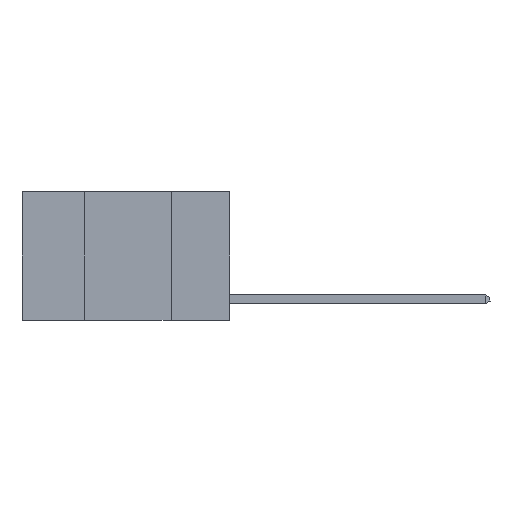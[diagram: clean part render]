
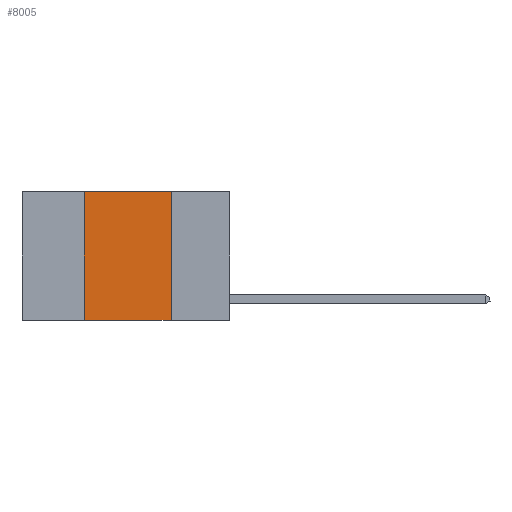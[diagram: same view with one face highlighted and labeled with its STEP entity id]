
A CAD part, left-side view. The second image highlights one B-rep face of the part: STEP entity #8005.
In plain terms, the highlighted planar face has unit normal (-1, 0, 0).
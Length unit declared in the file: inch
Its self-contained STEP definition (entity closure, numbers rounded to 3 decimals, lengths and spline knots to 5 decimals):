
#105 = CARTESIAN_POINT ( 'NONE',  ( 0., 0.6, -0.37 ) ) ;
#551 = CARTESIAN_POINT ( 'NONE',  ( 0., 0.42, -0.37 ) ) ;
#796 = CARTESIAN_POINT ( 'NONE',  ( 0., 0.6, 0. ) ) ;
#1732 = VERTEX_POINT ( 'NONE', #11590 ) ;
#1951 = VERTEX_POINT ( 'NONE', #7181 ) ;
#2041 = EDGE_CURVE ( 'NONE', #11272, #1732, #13572, .T. ) ;
#3205 = ORIENTED_EDGE ( 'NONE', *, *, #19679, .F. ) ;
#5479 = CARTESIAN_POINT ( 'NONE',  ( 0., 0.17, 0. ) ) ;
#6211 = CARTESIAN_POINT ( 'NONE',  ( 0., 0.42, 0. ) ) ;
#6630 = LINE ( 'NONE', #5479, #17073 ) ;
#7124 = VECTOR ( 'NONE', #17315, 39.37008 ) ;
#7181 = CARTESIAN_POINT ( 'NONE',  ( 0., 0.17, -0.37 ) ) ;
#8005 = ADVANCED_FACE ( 'NONE', ( #11233 ), #20389, .F. ) ;
#8915 = LINE ( 'NONE', #14596, #10787 ) ;
#10787 = VECTOR ( 'NONE', #16421, 39.37008 ) ;
#11227 = LINE ( 'NONE', #105, #19567 ) ;
#11233 = FACE_OUTER_BOUND ( 'NONE', #24631, .T. ) ;
#11272 = VERTEX_POINT ( 'NONE', #551 ) ;
#11290 = EDGE_CURVE ( 'NONE', #1732, #13888, #8915, .T. ) ;
#11547 = ORIENTED_EDGE ( 'NONE', *, *, #11290, .F. ) ;
#11590 = CARTESIAN_POINT ( 'NONE',  ( 0., 0.42, 0. ) ) ;
#12843 = EDGE_CURVE ( 'NONE', #11272, #1951, #11227, .T. ) ;
#13572 = LINE ( 'NONE', #6211, #7124 ) ;
#13888 = VERTEX_POINT ( 'NONE', #15855 ) ;
#14502 = DIRECTION ( 'NONE',  ( 1., 0., 0. ) ) ;
#14596 = CARTESIAN_POINT ( 'NONE',  ( 0., 0.6, 0. ) ) ;
#15855 = CARTESIAN_POINT ( 'NONE',  ( 0., 0.17, 0. ) ) ;
#16421 = DIRECTION ( 'NONE',  ( 0., -1., 0. ) ) ;
#16499 = DIRECTION ( 'NONE',  ( 0., 0., -1. ) ) ;
#16697 = ORIENTED_EDGE ( 'NONE', *, *, #2041, .F. ) ;
#17073 = VECTOR ( 'NONE', #17099, 39.37008 ) ;
#17099 = DIRECTION ( 'NONE',  ( 0., 0., -1. ) ) ;
#17187 = ORIENTED_EDGE ( 'NONE', *, *, #12843, .T. ) ;
#17315 = DIRECTION ( 'NONE',  ( 0., 0., 1. ) ) ;
#17714 = DIRECTION ( 'NONE',  ( 0., -1., 0. ) ) ;
#19567 = VECTOR ( 'NONE', #17714, 39.37008 ) ;
#19679 = EDGE_CURVE ( 'NONE', #13888, #1951, #6630, .T. ) ;
#20389 = PLANE ( 'NONE',  #21712 ) ;
#21712 = AXIS2_PLACEMENT_3D ( 'NONE', #796, #14502, #16499 ) ;
#24631 = EDGE_LOOP ( 'NONE', ( #3205, #11547, #16697, #17187 ) ) ;
